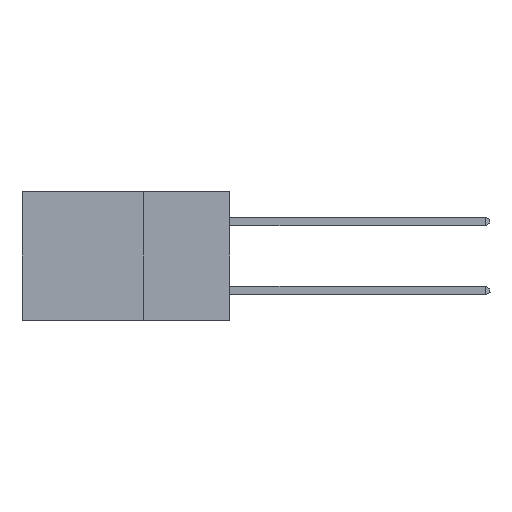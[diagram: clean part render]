
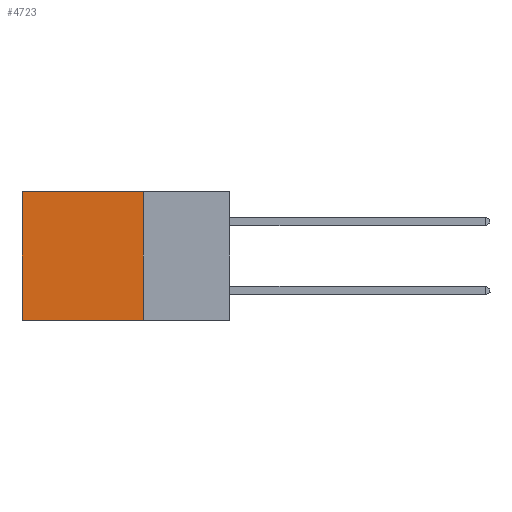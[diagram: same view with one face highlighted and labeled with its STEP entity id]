
A CAD part, left-side view. The second image highlights one B-rep face of the part: STEP entity #4723.
In plain terms, the highlighted planar face has unit normal (-1, 0, 0).
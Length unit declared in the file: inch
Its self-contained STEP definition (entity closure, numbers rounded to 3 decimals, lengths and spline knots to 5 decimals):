
#559 = VECTOR ( 'NONE', #5881, 39.37008 ) ;
#831 = EDGE_CURVE ( 'NONE', #5229, #12883, #19137, .T. ) ;
#1019 = VECTOR ( 'NONE', #3808, 39.37008 ) ;
#1918 = DIRECTION ( 'NONE',  ( 0., 0., -1. ) ) ;
#1977 = ORIENTED_EDGE ( 'NONE', *, *, #13021, .F. ) ;
#2047 = CARTESIAN_POINT ( 'NONE',  ( 0.298, 0.6, 0. ) ) ;
#2398 = LINE ( 'NONE', #19601, #16350 ) ;
#2803 = CARTESIAN_POINT ( 'NONE',  ( 0.298, 0.25, 0. ) ) ;
#2964 = CARTESIAN_POINT ( 'NONE',  ( 0.298, 0.25, 0. ) ) ;
#3808 = DIRECTION ( 'NONE',  ( 0., 0., -1. ) ) ;
#4337 = DIRECTION ( 'NONE',  ( 0., 1., 0. ) ) ;
#4723 = ADVANCED_FACE ( 'NONE', ( #13058 ), #10560, .F. ) ;
#5229 = VERTEX_POINT ( 'NONE', #13485 ) ;
#5400 = CARTESIAN_POINT ( 'NONE',  ( 0.298, 0.6, 0. ) ) ;
#5491 = CARTESIAN_POINT ( 'NONE',  ( 0.298, 0.6, -0.37 ) ) ;
#5881 = DIRECTION ( 'NONE',  ( 0., 0., -1. ) ) ;
#6904 = ORIENTED_EDGE ( 'NONE', *, *, #13925, .T. ) ;
#7555 = VECTOR ( 'NONE', #4337, 39.37008 ) ;
#7788 = LINE ( 'NONE', #5400, #1019 ) ;
#8694 = VERTEX_POINT ( 'NONE', #17493 ) ;
#8820 = EDGE_LOOP ( 'NONE', ( #6904, #17378, #1977, #15225 ) ) ;
#8833 = CARTESIAN_POINT ( 'NONE',  ( 0.298, 0.25, -0.37 ) ) ;
#10560 = PLANE ( 'NONE',  #17487 ) ;
#10954 = DIRECTION ( 'NONE',  ( 1., 0., 0. ) ) ;
#12869 = LINE ( 'NONE', #2803, #559 ) ;
#12883 = VERTEX_POINT ( 'NONE', #5491 ) ;
#13021 = EDGE_CURVE ( 'NONE', #8694, #5229, #12869, .T. ) ;
#13058 = FACE_OUTER_BOUND ( 'NONE', #8820, .T. ) ;
#13485 = CARTESIAN_POINT ( 'NONE',  ( 0.298, 0.25, -0.37 ) ) ;
#13622 = DIRECTION ( 'NONE',  ( 0., 1., 0. ) ) ;
#13925 = EDGE_CURVE ( 'NONE', #17712, #12883, #7788, .T. ) ;
#15225 = ORIENTED_EDGE ( 'NONE', *, *, #19098, .T. ) ;
#16350 = VECTOR ( 'NONE', #13622, 39.37008 ) ;
#17378 = ORIENTED_EDGE ( 'NONE', *, *, #831, .F. ) ;
#17487 = AXIS2_PLACEMENT_3D ( 'NONE', #2964, #10954, #1918 ) ;
#17493 = CARTESIAN_POINT ( 'NONE',  ( 0.298, 0.25, 0. ) ) ;
#17712 = VERTEX_POINT ( 'NONE', #2047 ) ;
#19098 = EDGE_CURVE ( 'NONE', #8694, #17712, #2398, .T. ) ;
#19137 = LINE ( 'NONE', #8833, #7555 ) ;
#19601 = CARTESIAN_POINT ( 'NONE',  ( 0.298, 0.25, 0. ) ) ;
